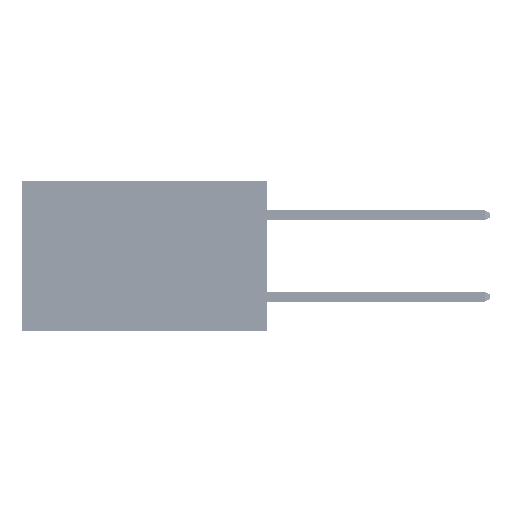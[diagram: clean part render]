
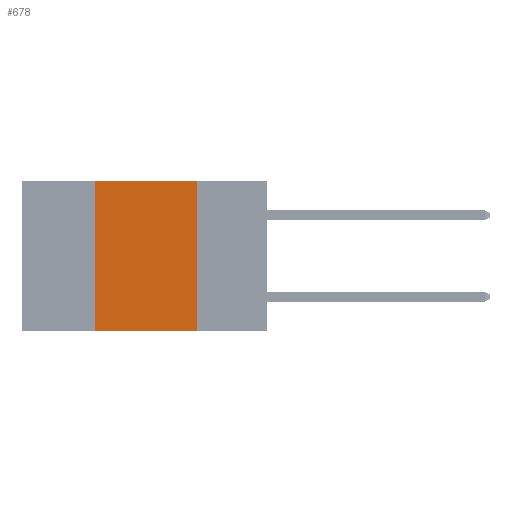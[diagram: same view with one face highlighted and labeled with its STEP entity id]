
A CAD part, left-side view. The second image highlights one B-rep face of the part: STEP entity #678.
In plain terms, the highlighted planar face has unit normal (-1, 0, 0).
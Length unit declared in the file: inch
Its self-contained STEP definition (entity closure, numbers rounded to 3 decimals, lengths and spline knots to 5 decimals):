
#540 = CARTESIAN_POINT ( 'NONE',  ( 0., 0.6, 0. ) ) ;
#617 = LINE ( 'NONE', #34898, #10636 ) ;
#678 = ADVANCED_FACE ( 'NONE', ( #41042 ), #24378, .F. ) ;
#6346 = VECTOR ( 'NONE', #21328, 39.37008 ) ;
#10295 = CARTESIAN_POINT ( 'NONE',  ( 0., 0.6, 0. ) ) ;
#10636 = VECTOR ( 'NONE', #15084, 39.37008 ) ;
#10873 = EDGE_CURVE ( 'NONE', #28635, #43043, #11537, .T. ) ;
#11316 = DIRECTION ( 'NONE',  ( 0., -1., 0. ) ) ;
#11537 = LINE ( 'NONE', #26748, #43457 ) ;
#12630 = VERTEX_POINT ( 'NONE', #33897 ) ;
#14527 = LINE ( 'NONE', #38371, #6346 ) ;
#14689 = DIRECTION ( 'NONE',  ( 0., -1., 0. ) ) ;
#15084 = DIRECTION ( 'NONE',  ( 0., 0., -1. ) ) ;
#18880 = EDGE_CURVE ( 'NONE', #28635, #12630, #14527, .T. ) ;
#21328 = DIRECTION ( 'NONE',  ( 0., 0., 1. ) ) ;
#21380 = AXIS2_PLACEMENT_3D ( 'NONE', #540, #48209, #36472 ) ;
#23001 = LINE ( 'NONE', #10295, #38714 ) ;
#24378 = PLANE ( 'NONE',  #21380 ) ;
#25160 = CARTESIAN_POINT ( 'NONE',  ( 0., 0.17, 0. ) ) ;
#25232 = EDGE_CURVE ( 'NONE', #41540, #43043, #617, .T. ) ;
#26748 = CARTESIAN_POINT ( 'NONE',  ( 0., 0.6, -0.37 ) ) ;
#28635 = VERTEX_POINT ( 'NONE', #43768 ) ;
#32472 = ORIENTED_EDGE ( 'NONE', *, *, #45752, .F. ) ;
#33897 = CARTESIAN_POINT ( 'NONE',  ( 0., 0.42, 0. ) ) ;
#34310 = ORIENTED_EDGE ( 'NONE', *, *, #10873, .T. ) ;
#34898 = CARTESIAN_POINT ( 'NONE',  ( 0., 0.17, 0. ) ) ;
#36472 = DIRECTION ( 'NONE',  ( 0., 0., -1. ) ) ;
#38371 = CARTESIAN_POINT ( 'NONE',  ( 0., 0.42, 0. ) ) ;
#38714 = VECTOR ( 'NONE', #14689, 39.37008 ) ;
#40786 = EDGE_LOOP ( 'NONE', ( #47739, #32472, #50524, #34310 ) ) ;
#41042 = FACE_OUTER_BOUND ( 'NONE', #40786, .T. ) ;
#41540 = VERTEX_POINT ( 'NONE', #25160 ) ;
#43043 = VERTEX_POINT ( 'NONE', #51188 ) ;
#43457 = VECTOR ( 'NONE', #11316, 39.37008 ) ;
#43768 = CARTESIAN_POINT ( 'NONE',  ( 0., 0.42, -0.37 ) ) ;
#45752 = EDGE_CURVE ( 'NONE', #12630, #41540, #23001, .T. ) ;
#47739 = ORIENTED_EDGE ( 'NONE', *, *, #25232, .F. ) ;
#48209 = DIRECTION ( 'NONE',  ( 1., 0., 0. ) ) ;
#50524 = ORIENTED_EDGE ( 'NONE', *, *, #18880, .F. ) ;
#51188 = CARTESIAN_POINT ( 'NONE',  ( 0., 0.17, -0.37 ) ) ;
